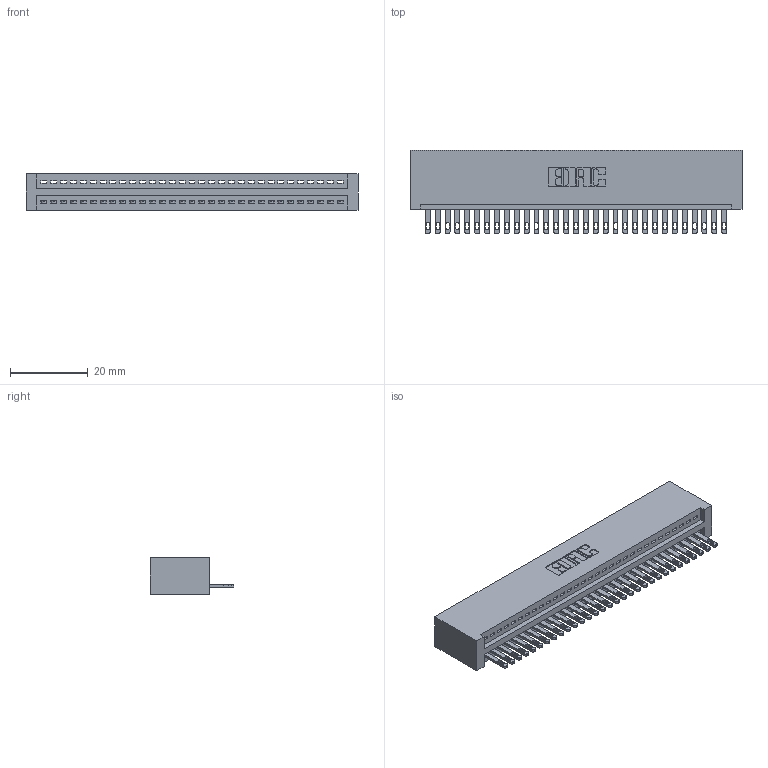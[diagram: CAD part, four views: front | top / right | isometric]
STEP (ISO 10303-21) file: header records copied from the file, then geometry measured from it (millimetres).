
FILE_DESCRIPTION (( 'STEP AP203' ), '1' );
FILE_NAME ('895-031-500-101.STEP', '2020-09-25T18:34:44', ( '' ), ( '' ), 'SwSTEP 2.0', 'SolidWorks 2020', '' );
FILE_SCHEMA (( 'CONFIG_CONTROL_DESIGN' ));
Length unit declared in the file: inch
Products named in the file (3): 845 Part_No Mounting Lugs; 345-292-001_345-293-100; 895-031-500-101
Assembly tree (32 placements, depth 2):
  895-031-500-101
    845 Part_No Mounting Lugs
    345-292-001_345-293-100  x31
Bounding box: 85.34 x 21.51 x 9.4 mm (x, y, z)
Volume: 8619.5 mm3; surface area: 11564.8 mm2
Topology: 32 solids, 32 shells, 1792 faces, 5525 edges, 3682 vertices
Faces by surface type: plane 1130, cylinder 662
Entity records: 24465 total; most frequent: CARTESIAN_POINT 4245, ORIENTED_EDGE 4210, DIRECTION 3719, EDGE_CURVE 2105, VECTOR 1853, LINE 1853, VERTEX_POINT 1402, AXIS2_PLACEMENT_3D 933
